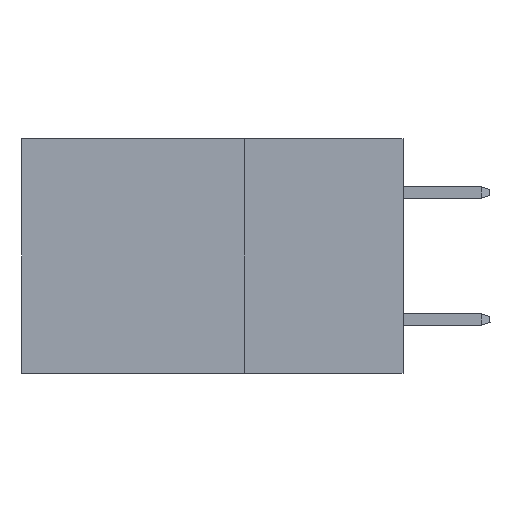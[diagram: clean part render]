
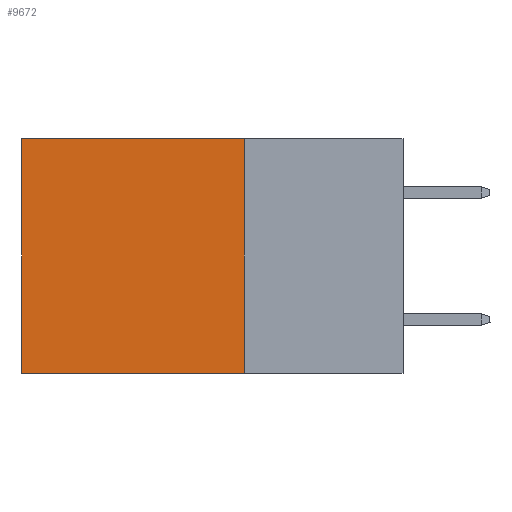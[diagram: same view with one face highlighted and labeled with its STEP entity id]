
A CAD part, left-side view. The second image highlights one B-rep face of the part: STEP entity #9672.
In plain terms, the highlighted planar face has unit normal (-1, 0, 0).
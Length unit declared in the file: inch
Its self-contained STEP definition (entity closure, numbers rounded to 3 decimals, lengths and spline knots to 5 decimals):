
#36 = CARTESIAN_POINT ( 'NONE',  ( 0.2875, 0.6, 0. ) ) ;
#38 = CARTESIAN_POINT ( 'NONE',  ( 0.2875, 0.6, -0.37 ) ) ;
#306 = DIRECTION ( 'NONE',  ( 0., 1., 0. ) ) ;
#362 = CARTESIAN_POINT ( 'NONE',  ( 0.2875, 0.25, -0.37 ) ) ;
#458 = CARTESIAN_POINT ( 'NONE',  ( 0.2875, 0.6, 0. ) ) ;
#499 = CARTESIAN_POINT ( 'NONE',  ( 0.2875, 0.25, 0. ) ) ;
#619 = EDGE_LOOP ( 'NONE', ( #3837, #4001, #11146, #3338 ) ) ;
#1179 = EDGE_CURVE ( 'NONE', #4584, #7863, #3486, .T. ) ;
#2524 = LINE ( 'NONE', #9002, #4350 ) ;
#2764 = VECTOR ( 'NONE', #306, 39.37008 ) ;
#3338 = ORIENTED_EDGE ( 'NONE', *, *, #1179, .T. ) ;
#3465 = EDGE_CURVE ( 'NONE', #4584, #10964, #2524, .T. ) ;
#3486 = LINE ( 'NONE', #9257, #8726 ) ;
#3829 = EDGE_CURVE ( 'NONE', #10964, #10944, #9028, .T. ) ;
#3837 = ORIENTED_EDGE ( 'NONE', *, *, #8823, .T. ) ;
#4001 = ORIENTED_EDGE ( 'NONE', *, *, #3829, .F. ) ;
#4279 = DIRECTION ( 'NONE',  ( 1., 0., 0. ) ) ;
#4350 = VECTOR ( 'NONE', #8122, 39.37008 ) ;
#4584 = VERTEX_POINT ( 'NONE', #7891 ) ;
#4691 = LINE ( 'NONE', #36, #5412 ) ;
#5220 = FACE_OUTER_BOUND ( 'NONE', #619, .T. ) ;
#5412 = VECTOR ( 'NONE', #10334, 39.37008 ) ;
#7462 = CARTESIAN_POINT ( 'NONE',  ( 0.2875, 0.25, -0.37 ) ) ;
#7863 = VERTEX_POINT ( 'NONE', #458 ) ;
#7891 = CARTESIAN_POINT ( 'NONE',  ( 0.2875, 0.25, 0. ) ) ;
#8122 = DIRECTION ( 'NONE',  ( 0., 0., -1. ) ) ;
#8726 = VECTOR ( 'NONE', #11060, 39.37008 ) ;
#8823 = EDGE_CURVE ( 'NONE', #7863, #10944, #4691, .T. ) ;
#8998 = PLANE ( 'NONE',  #9581 ) ;
#9002 = CARTESIAN_POINT ( 'NONE',  ( 0.2875, 0.25, 0. ) ) ;
#9028 = LINE ( 'NONE', #362, #2764 ) ;
#9257 = CARTESIAN_POINT ( 'NONE',  ( 0.2875, 0.25, 0. ) ) ;
#9581 = AXIS2_PLACEMENT_3D ( 'NONE', #499, #4279, #9983 ) ;
#9672 = ADVANCED_FACE ( 'NONE', ( #5220 ), #8998, .F. ) ;
#9983 = DIRECTION ( 'NONE',  ( 0., 0., -1. ) ) ;
#10334 = DIRECTION ( 'NONE',  ( 0., 0., -1. ) ) ;
#10944 = VERTEX_POINT ( 'NONE', #38 ) ;
#10964 = VERTEX_POINT ( 'NONE', #7462 ) ;
#11060 = DIRECTION ( 'NONE',  ( 0., 1., 0. ) ) ;
#11146 = ORIENTED_EDGE ( 'NONE', *, *, #3465, .F. ) ;
